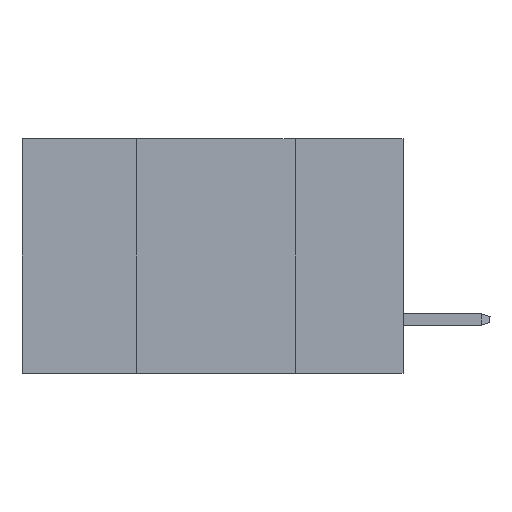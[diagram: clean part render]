
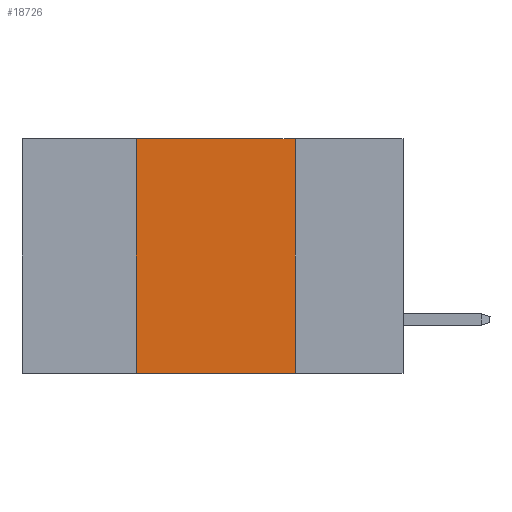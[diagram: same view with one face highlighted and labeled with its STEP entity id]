
A CAD part, left-side view. The second image highlights one B-rep face of the part: STEP entity #18726.
In plain terms, the highlighted planar face has unit normal (-1, 0, 0).
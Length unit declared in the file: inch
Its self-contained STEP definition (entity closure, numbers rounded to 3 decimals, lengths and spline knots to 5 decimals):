
#1 = CARTESIAN_POINT ( 'NONE',  ( 0., 0.42, 0. ) ) ;
#694 = ORIENTED_EDGE ( 'NONE', *, *, #12542, .T. ) ;
#773 = AXIS2_PLACEMENT_3D ( 'NONE', #18631, #22622, #22893 ) ;
#1886 = DIRECTION ( 'NONE',  ( 0., 0., -1. ) ) ;
#2073 = LINE ( 'NONE', #1, #10244 ) ;
#2772 = FACE_OUTER_BOUND ( 'NONE', #10786, .T. ) ;
#3088 = EDGE_CURVE ( 'NONE', #22337, #18333, #2073, .T. ) ;
#5074 = CARTESIAN_POINT ( 'NONE',  ( 0., 0.6, -0.37 ) ) ;
#5383 = CARTESIAN_POINT ( 'NONE',  ( 0., 0.42, 0. ) ) ;
#5630 = DIRECTION ( 'NONE',  ( 0., -1., 0. ) ) ;
#6154 = ORIENTED_EDGE ( 'NONE', *, *, #10512, .F. ) ;
#6214 = VECTOR ( 'NONE', #5630, 39.37008 ) ;
#7615 = VERTEX_POINT ( 'NONE', #15586 ) ;
#7856 = ORIENTED_EDGE ( 'NONE', *, *, #11859, .F. ) ;
#7907 = DIRECTION ( 'NONE',  ( 0., 0., 1. ) ) ;
#8099 = CARTESIAN_POINT ( 'NONE',  ( 0., 0.17, 0. ) ) ;
#9092 = DIRECTION ( 'NONE',  ( 0., -1., 0. ) ) ;
#9934 = VECTOR ( 'NONE', #1886, 39.37008 ) ;
#10244 = VECTOR ( 'NONE', #7907, 39.37008 ) ;
#10512 = EDGE_CURVE ( 'NONE', #18333, #7615, #25458, .T. ) ;
#10532 = PLANE ( 'NONE',  #773 ) ;
#10773 = VECTOR ( 'NONE', #9092, 39.37008 ) ;
#10786 = EDGE_LOOP ( 'NONE', ( #7856, #6154, #24977, #694 ) ) ;
#11853 = LINE ( 'NONE', #8099, #9934 ) ;
#11859 = EDGE_CURVE ( 'NONE', #7615, #14124, #11853, .T. ) ;
#12542 = EDGE_CURVE ( 'NONE', #22337, #14124, #16904, .T. ) ;
#14124 = VERTEX_POINT ( 'NONE', #25085 ) ;
#15586 = CARTESIAN_POINT ( 'NONE',  ( 0., 0.17, 0. ) ) ;
#16904 = LINE ( 'NONE', #5074, #10773 ) ;
#18333 = VERTEX_POINT ( 'NONE', #5383 ) ;
#18631 = CARTESIAN_POINT ( 'NONE',  ( 0., 0.6, 0. ) ) ;
#18726 = ADVANCED_FACE ( 'NONE', ( #2772 ), #10532, .F. ) ;
#19823 = CARTESIAN_POINT ( 'NONE',  ( 0., 0.6, 0. ) ) ;
#22337 = VERTEX_POINT ( 'NONE', #25105 ) ;
#22622 = DIRECTION ( 'NONE',  ( 1., 0., 0. ) ) ;
#22893 = DIRECTION ( 'NONE',  ( 0., 0., -1. ) ) ;
#24977 = ORIENTED_EDGE ( 'NONE', *, *, #3088, .F. ) ;
#25085 = CARTESIAN_POINT ( 'NONE',  ( 0., 0.17, -0.37 ) ) ;
#25105 = CARTESIAN_POINT ( 'NONE',  ( 0., 0.42, -0.37 ) ) ;
#25458 = LINE ( 'NONE', #19823, #6214 ) ;
